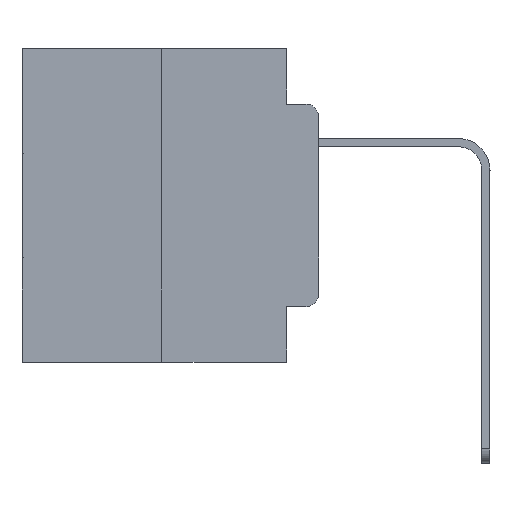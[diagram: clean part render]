
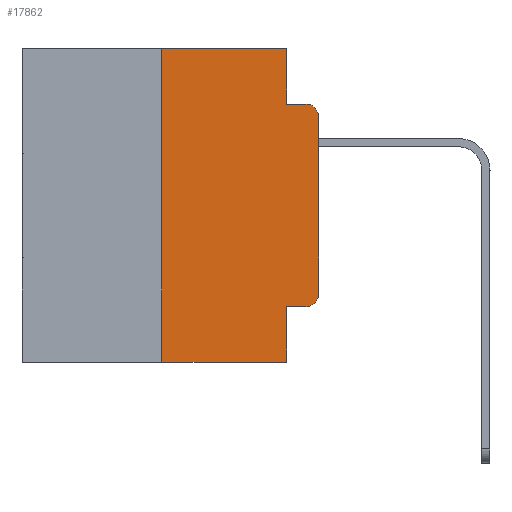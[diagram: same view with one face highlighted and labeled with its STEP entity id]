
A CAD part, left-side view. The second image highlights one B-rep face of the part: STEP entity #17862.
In plain terms, the highlighted planar face has unit normal (-1, 0, 0).
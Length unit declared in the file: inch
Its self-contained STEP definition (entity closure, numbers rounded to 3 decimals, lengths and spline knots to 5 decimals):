
#162 = ORIENTED_EDGE ( 'NONE', *, *, #3423, .F. ) ;
#329 = DIRECTION ( 'NONE',  ( 0., 0., -1. ) ) ;
#652 = CARTESIAN_POINT ( 'NONE',  ( 0., 0.051, -0.4115 ) ) ;
#699 = CARTESIAN_POINT ( 'NONE',  ( 0., 0.25, 0. ) ) ;
#1070 = CARTESIAN_POINT ( 'NONE',  ( 0., 0., -0.1085 ) ) ;
#1436 = CARTESIAN_POINT ( 'NONE',  ( 0., 0.473, -0.5 ) ) ;
#1639 = CARTESIAN_POINT ( 'NONE',  ( 0., 0., -0.3915 ) ) ;
#1661 = VECTOR ( 'NONE', #16511, 39.37008 ) ;
#2972 = VECTOR ( 'NONE', #26187, 39.37008 ) ;
#3423 = EDGE_CURVE ( 'NONE', #19549, #15262, #17073, .T. ) ;
#3616 = FACE_OUTER_BOUND ( 'NONE', #12979, .T. ) ;
#3757 = ORIENTED_EDGE ( 'NONE', *, *, #17336, .T. ) ;
#4520 = CARTESIAN_POINT ( 'NONE',  ( 0., 0.051, -0.0885 ) ) ;
#4702 = VERTEX_POINT ( 'NONE', #9051 ) ;
#5266 = ORIENTED_EDGE ( 'NONE', *, *, #5968, .F. ) ;
#5968 = EDGE_CURVE ( 'NONE', #10028, #19549, #12913, .T. ) ;
#6469 = ORIENTED_EDGE ( 'NONE', *, *, #20753, .T. ) ;
#6816 = VECTOR ( 'NONE', #25859, 39.37008 ) ;
#7175 = EDGE_CURVE ( 'NONE', #10326, #25417, #20857, .T. ) ;
#7214 = CIRCLE ( 'NONE', #9372, 0.02 ) ;
#8700 = VECTOR ( 'NONE', #16211, 39.37008 ) ;
#8736 = VERTEX_POINT ( 'NONE', #14221 ) ;
#8871 = ORIENTED_EDGE ( 'NONE', *, *, #20769, .F. ) ;
#9051 = CARTESIAN_POINT ( 'NONE',  ( 0., 0.02, -0.0885 ) ) ;
#9085 = EDGE_CURVE ( 'NONE', #26576, #4702, #25664, .T. ) ;
#9372 = AXIS2_PLACEMENT_3D ( 'NONE', #20927, #23238, #27380 ) ;
#9380 = LINE ( 'NONE', #652, #17389 ) ;
#10028 = VERTEX_POINT ( 'NONE', #25988 ) ;
#10174 = EDGE_CURVE ( 'NONE', #8736, #10326, #24618, .T. ) ;
#10273 = CARTESIAN_POINT ( 'NONE',  ( 0., 0.051, 0. ) ) ;
#10326 = VERTEX_POINT ( 'NONE', #1639 ) ;
#11032 = PLANE ( 'NONE',  #16135 ) ;
#11518 = CARTESIAN_POINT ( 'NONE',  ( 0., 0.051, -0.0885 ) ) ;
#11670 = CARTESIAN_POINT ( 'NONE',  ( 0., 0.051, -0.5 ) ) ;
#12216 = LINE ( 'NONE', #27286, #20898 ) ;
#12245 = DIRECTION ( 'NONE',  ( 0., 0., -1. ) ) ;
#12913 = LINE ( 'NONE', #699, #20270 ) ;
#12914 = AXIS2_PLACEMENT_3D ( 'NONE', #20391, #18143, #15827 ) ;
#12979 = EDGE_LOOP ( 'NONE', ( #25927, #6469, #16046, #23278, #162, #5266, #19751, #8871, #3757, #18620 ) ) ;
#13187 = DIRECTION ( 'NONE',  ( 1., 0., 0. ) ) ;
#14067 = EDGE_CURVE ( 'NONE', #10028, #21161, #19782, .T. ) ;
#14221 = CARTESIAN_POINT ( 'NONE',  ( 0., 0.02, -0.4115 ) ) ;
#15262 = VERTEX_POINT ( 'NONE', #10273 ) ;
#15747 = LINE ( 'NONE', #18435, #8700 ) ;
#15827 = DIRECTION ( 'NONE',  ( 0., 0., -1. ) ) ;
#16046 = ORIENTED_EDGE ( 'NONE', *, *, #9085, .F. ) ;
#16135 = AXIS2_PLACEMENT_3D ( 'NONE', #25973, #13187, #329 ) ;
#16211 = DIRECTION ( 'NONE',  ( 0., 0., -1. ) ) ;
#16511 = DIRECTION ( 'NONE',  ( 0., -1., 0. ) ) ;
#17073 = LINE ( 'NONE', #25424, #2972 ) ;
#17336 = EDGE_CURVE ( 'NONE', #22684, #8736, #9380, .T. ) ;
#17389 = VECTOR ( 'NONE', #24668, 39.37008 ) ;
#17400 = EDGE_CURVE ( 'NONE', #15262, #26576, #15747, .T. ) ;
#17454 = CARTESIAN_POINT ( 'NONE',  ( 0., 0., 0. ) ) ;
#17862 = ADVANCED_FACE ( 'NONE', ( #3616 ), #11032, .F. ) ;
#18143 = DIRECTION ( 'NONE',  ( -1., 0., 0. ) ) ;
#18435 = CARTESIAN_POINT ( 'NONE',  ( 0., 0.051, 0. ) ) ;
#18620 = ORIENTED_EDGE ( 'NONE', *, *, #10174, .T. ) ;
#19500 = DIRECTION ( 'NONE',  ( 0., -1., 0. ) ) ;
#19549 = VERTEX_POINT ( 'NONE', #23125 ) ;
#19751 = ORIENTED_EDGE ( 'NONE', *, *, #14067, .T. ) ;
#19782 = LINE ( 'NONE', #1436, #1661 ) ;
#20270 = VECTOR ( 'NONE', #21761, 39.37008 ) ;
#20391 = CARTESIAN_POINT ( 'NONE',  ( 0., 0.02, -0.3915 ) ) ;
#20753 = EDGE_CURVE ( 'NONE', #25417, #4702, #7214, .T. ) ;
#20769 = EDGE_CURVE ( 'NONE', #22684, #21161, #12216, .T. ) ;
#20857 = LINE ( 'NONE', #17454, #6816 ) ;
#20898 = VECTOR ( 'NONE', #12245, 39.37008 ) ;
#20927 = CARTESIAN_POINT ( 'NONE',  ( 0., 0.02, -0.1085 ) ) ;
#21161 = VERTEX_POINT ( 'NONE', #11670 ) ;
#21761 = DIRECTION ( 'NONE',  ( 0., 0., 1. ) ) ;
#22684 = VERTEX_POINT ( 'NONE', #25657 ) ;
#23125 = CARTESIAN_POINT ( 'NONE',  ( 0., 0.25, 0. ) ) ;
#23238 = DIRECTION ( 'NONE',  ( -1., 0., 0. ) ) ;
#23278 = ORIENTED_EDGE ( 'NONE', *, *, #17400, .F. ) ;
#23610 = VECTOR ( 'NONE', #19500, 39.37008 ) ;
#24618 = CIRCLE ( 'NONE', #12914, 0.02 ) ;
#24668 = DIRECTION ( 'NONE',  ( 0., -1., 0. ) ) ;
#25417 = VERTEX_POINT ( 'NONE', #1070 ) ;
#25424 = CARTESIAN_POINT ( 'NONE',  ( 0., 0.473, 0. ) ) ;
#25657 = CARTESIAN_POINT ( 'NONE',  ( 0., 0.051, -0.4115 ) ) ;
#25664 = LINE ( 'NONE', #4520, #23610 ) ;
#25859 = DIRECTION ( 'NONE',  ( 0., 0., 1. ) ) ;
#25927 = ORIENTED_EDGE ( 'NONE', *, *, #7175, .T. ) ;
#25973 = CARTESIAN_POINT ( 'NONE',  ( 0., 0.473, 0. ) ) ;
#25988 = CARTESIAN_POINT ( 'NONE',  ( 0., 0.25, -0.5 ) ) ;
#26187 = DIRECTION ( 'NONE',  ( 0., -1., 0. ) ) ;
#26576 = VERTEX_POINT ( 'NONE', #11518 ) ;
#27286 = CARTESIAN_POINT ( 'NONE',  ( 0., 0.051, 0. ) ) ;
#27380 = DIRECTION ( 'NONE',  ( 0., 0., -1. ) ) ;
